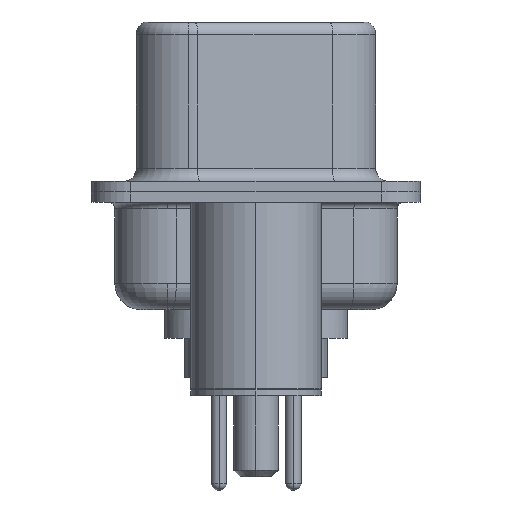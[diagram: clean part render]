
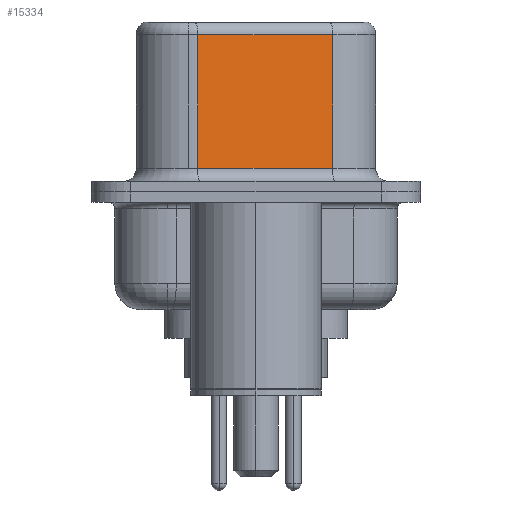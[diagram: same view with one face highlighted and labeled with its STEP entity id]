
A CAD part, left-side view. The second image highlights one B-rep face of the part: STEP entity #15334.
In plain terms, the highlighted planar face has unit normal (-0.985, -0.174, 0).
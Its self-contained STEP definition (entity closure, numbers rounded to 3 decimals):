
#971 = VECTOR ( 'NONE', #12716, 1000. ) ;
#1488 = VERTEX_POINT ( 'NONE', #15116 ) ;
#1891 = PLANE ( 'NONE',  #1925 ) ;
#1925 = AXIS2_PLACEMENT_3D ( 'NONE', #11776, #20106, #10211 ) ;
#4356 = EDGE_CURVE ( 'NONE', #5291, #17120, #17234, .T. ) ;
#4369 = ORIENTED_EDGE ( 'NONE', *, *, #4356, .F. ) ;
#5291 = VERTEX_POINT ( 'NONE', #12043 ) ;
#5453 = VECTOR ( 'NONE', #21322, 1000. ) ;
#7755 = CARTESIAN_POINT ( 'NONE',  ( 4.585, -2.927, 6.02 ) ) ;
#8499 = VECTOR ( 'NONE', #12883, 1000. ) ;
#9611 = DIRECTION ( 'NONE',  ( 0.174, -0.985, 0. ) ) ;
#9885 = LINE ( 'NONE', #17892, #5453 ) ;
#10081 = FACE_OUTER_BOUND ( 'NONE', #21203, .T. ) ;
#10211 = DIRECTION ( 'NONE',  ( -0.174, 0.985, 0. ) ) ;
#10283 = EDGE_CURVE ( 'NONE', #16743, #17120, #19684, .T. ) ;
#11216 = CARTESIAN_POINT ( 'NONE',  ( 3.675, 2.233, 0.9 ) ) ;
#11404 = VECTOR ( 'NONE', #9611, 1000. ) ;
#11776 = CARTESIAN_POINT ( 'NONE',  ( 4.585, -2.927, 6.52 ) ) ;
#12043 = CARTESIAN_POINT ( 'NONE',  ( 4.585, -2.927, 6.02 ) ) ;
#12716 = DIRECTION ( 'NONE',  ( -0.174, 0.985, 0. ) ) ;
#12883 = DIRECTION ( 'NONE',  ( 0., 0., -1. ) ) ;
#13851 = EDGE_CURVE ( 'NONE', #1488, #16743, #9885, .T. ) ;
#14951 = ORIENTED_EDGE ( 'NONE', *, *, #18288, .T. ) ;
#15116 = CARTESIAN_POINT ( 'NONE',  ( 3.675, 2.233, 6.02 ) ) ;
#15334 = ADVANCED_FACE ( 'NONE', ( #10081 ), #1891, .F. ) ;
#15739 = ORIENTED_EDGE ( 'NONE', *, *, #13851, .T. ) ;
#16743 = VERTEX_POINT ( 'NONE', #11216 ) ;
#16834 = CARTESIAN_POINT ( 'NONE',  ( 4.585, -2.927, 0.9 ) ) ;
#17120 = VERTEX_POINT ( 'NONE', #16834 ) ;
#17234 = LINE ( 'NONE', #19550, #8499 ) ;
#17892 = CARTESIAN_POINT ( 'NONE',  ( 3.675, 2.233, 6.52 ) ) ;
#18288 = EDGE_CURVE ( 'NONE', #5291, #1488, #18510, .T. ) ;
#18510 = LINE ( 'NONE', #7755, #971 ) ;
#18634 = ORIENTED_EDGE ( 'NONE', *, *, #10283, .T. ) ;
#19550 = CARTESIAN_POINT ( 'NONE',  ( 4.585, -2.927, 6.52 ) ) ;
#19684 = LINE ( 'NONE', #21159, #11404 ) ;
#20106 = DIRECTION ( 'NONE',  ( 0.985, 0.174, 0. ) ) ;
#21159 = CARTESIAN_POINT ( 'NONE',  ( 4.585, -2.927, 0.9 ) ) ;
#21203 = EDGE_LOOP ( 'NONE', ( #4369, #14951, #15739, #18634 ) ) ;
#21322 = DIRECTION ( 'NONE',  ( 0., 0., -1. ) ) ;
